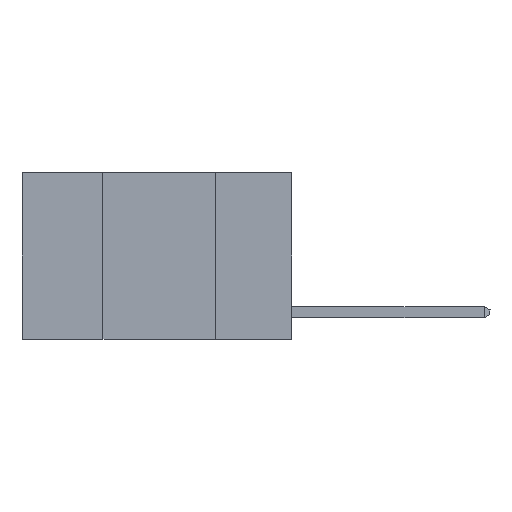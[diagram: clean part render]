
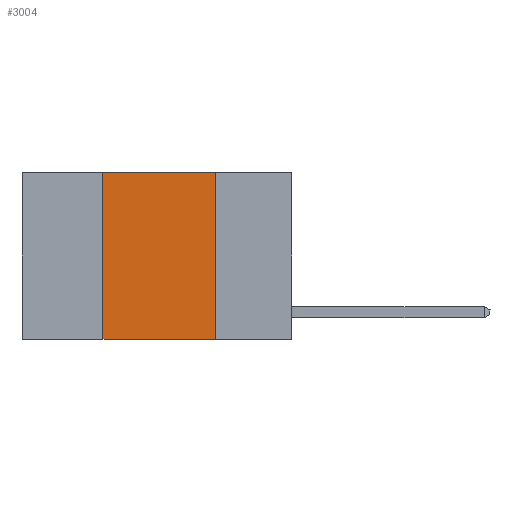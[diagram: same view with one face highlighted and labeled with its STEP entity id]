
A CAD part, left-side view. The second image highlights one B-rep face of the part: STEP entity #3004.
In plain terms, the highlighted planar face has unit normal (-1, 0, 0).
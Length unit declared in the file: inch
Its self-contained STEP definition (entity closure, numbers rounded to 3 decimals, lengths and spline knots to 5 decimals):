
#67 = VECTOR ( 'NONE', #7437, 39.37008 ) ;
#84 = VERTEX_POINT ( 'NONE', #19497 ) ;
#500 = VERTEX_POINT ( 'NONE', #6780 ) ;
#2616 = VECTOR ( 'NONE', #22018, 39.37008 ) ;
#3004 = ADVANCED_FACE ( 'NONE', ( #23203 ), #9814, .F. ) ;
#3516 = VECTOR ( 'NONE', #14010, 39.37008 ) ;
#3558 = ORIENTED_EDGE ( 'NONE', *, *, #24253, .F. ) ;
#6060 = EDGE_CURVE ( 'NONE', #84, #10972, #25434, .T. ) ;
#6780 = CARTESIAN_POINT ( 'NONE',  ( 0., 0.42, 0. ) ) ;
#7437 = DIRECTION ( 'NONE',  ( 0., 0., 1. ) ) ;
#7651 = EDGE_CURVE ( 'NONE', #18125, #10972, #13860, .T. ) ;
#8995 = VECTOR ( 'NONE', #23392, 39.37008 ) ;
#9668 = CARTESIAN_POINT ( 'NONE',  ( 0., 0.6, 0. ) ) ;
#9733 = CARTESIAN_POINT ( 'NONE',  ( 0., 0.6, 0. ) ) ;
#9814 = PLANE ( 'NONE',  #12385 ) ;
#10972 = VERTEX_POINT ( 'NONE', #21088 ) ;
#11913 = DIRECTION ( 'NONE',  ( 0., 0., -1. ) ) ;
#12385 = AXIS2_PLACEMENT_3D ( 'NONE', #9733, #24223, #11913 ) ;
#12562 = EDGE_LOOP ( 'NONE', ( #19394, #3558, #20692, #26105 ) ) ;
#13860 = LINE ( 'NONE', #15211, #8995 ) ;
#14010 = DIRECTION ( 'NONE',  ( 0., -1., 0. ) ) ;
#15211 = CARTESIAN_POINT ( 'NONE',  ( 0., 0.17, 0. ) ) ;
#18125 = VERTEX_POINT ( 'NONE', #21928 ) ;
#18451 = LINE ( 'NONE', #9668, #2616 ) ;
#19394 = ORIENTED_EDGE ( 'NONE', *, *, #7651, .F. ) ;
#19497 = CARTESIAN_POINT ( 'NONE',  ( 0., 0.42, -0.37 ) ) ;
#20692 = ORIENTED_EDGE ( 'NONE', *, *, #23042, .F. ) ;
#21088 = CARTESIAN_POINT ( 'NONE',  ( 0., 0.17, -0.37 ) ) ;
#21928 = CARTESIAN_POINT ( 'NONE',  ( 0., 0.17, 0. ) ) ;
#22018 = DIRECTION ( 'NONE',  ( 0., -1., 0. ) ) ;
#22068 = LINE ( 'NONE', #23935, #67 ) ;
#23042 = EDGE_CURVE ( 'NONE', #84, #500, #22068, .T. ) ;
#23203 = FACE_OUTER_BOUND ( 'NONE', #12562, .T. ) ;
#23392 = DIRECTION ( 'NONE',  ( 0., 0., -1. ) ) ;
#23935 = CARTESIAN_POINT ( 'NONE',  ( 0., 0.42, 0. ) ) ;
#24223 = DIRECTION ( 'NONE',  ( 1., 0., 0. ) ) ;
#24230 = CARTESIAN_POINT ( 'NONE',  ( 0., 0.6, -0.37 ) ) ;
#24253 = EDGE_CURVE ( 'NONE', #500, #18125, #18451, .T. ) ;
#25434 = LINE ( 'NONE', #24230, #3516 ) ;
#26105 = ORIENTED_EDGE ( 'NONE', *, *, #6060, .T. ) ;
